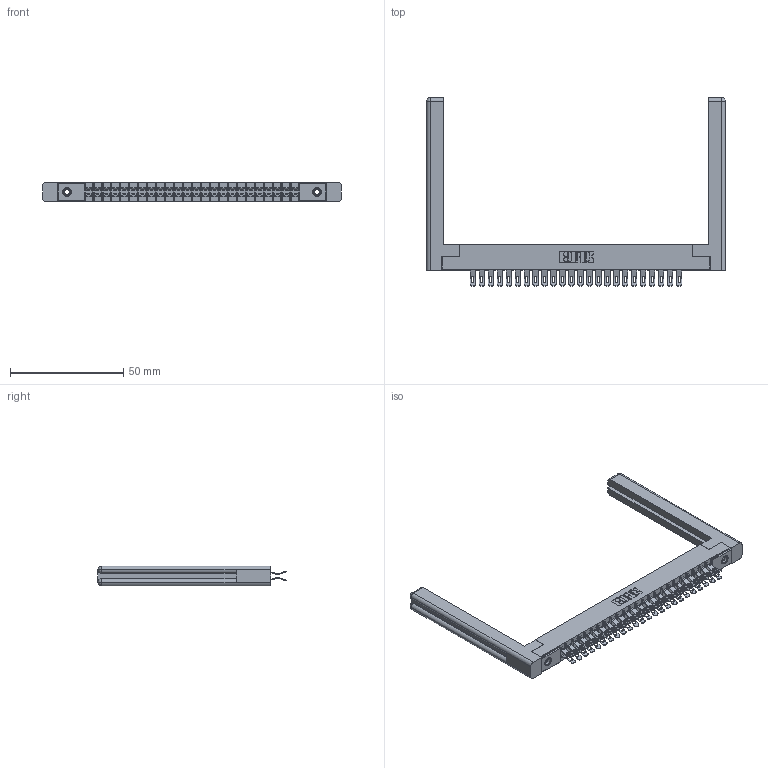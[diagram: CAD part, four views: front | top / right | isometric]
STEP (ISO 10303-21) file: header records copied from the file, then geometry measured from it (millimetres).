
FILE_DESCRIPTION (( 'STEP AP203' ), '1' );
FILE_NAME ('305-048-555-558.STEP', '2019-09-09T21:19:42', ( '' ), ( '' ), 'SwSTEP 2.0', 'SolidWorks 2016', '' );
FILE_SCHEMA (( 'CONFIG_CONTROL_DESIGN' ));
Length unit declared in the file: inch
Products named in the file (5): 307-220-058; 345-250-001_345-250-001-102; 305-048-555-558; 305-290-001_555; 305 Part_.156 Dia
Assembly tree (53 placements, depth 2):
  305-048-555-558
    305 Part_.156 Dia
    305-290-001_555  x48
    345-250-001_345-250-001-102  x2
    307-220-058  x2
Bounding box: 131.72 x 83.06 x 8.71 mm (x, y, z)
Volume: 15788.7 mm3; surface area: 21957.8 mm2
Topology: 53 solids, 53 shells, 3426 faces, 10150 edges, 6624 vertices
Faces by surface type: plane 1688, cylinder 1618, sphere 96, cone 12, torus 12
Entity records: 31434 total; most frequent: CARTESIAN_POINT 5235, ORIENTED_EDGE 5126, DIRECTION 5035, EDGE_CURVE 2563, LINE 2023, VECTOR 2023, VERTEX_POINT 1636, AXIS2_PLACEMENT_3D 1506
